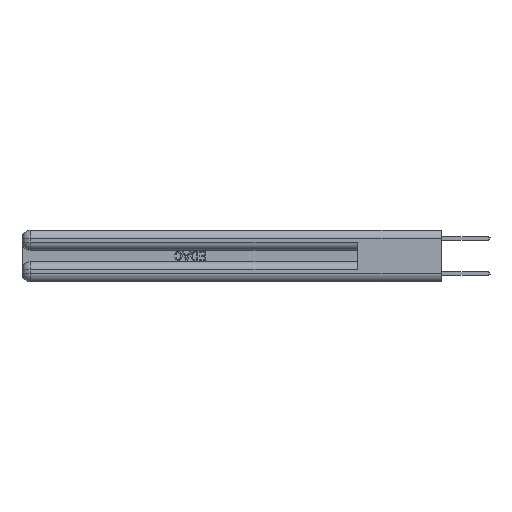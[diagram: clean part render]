
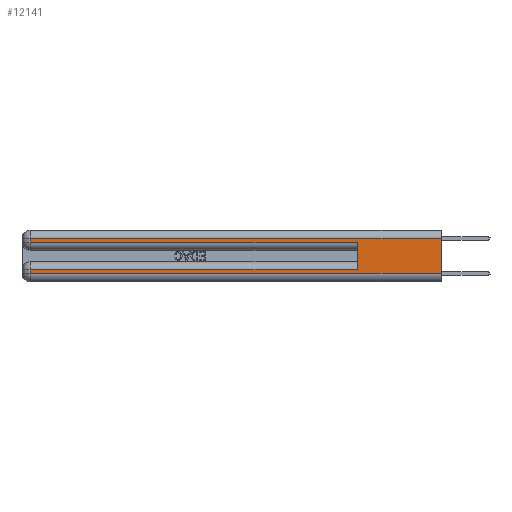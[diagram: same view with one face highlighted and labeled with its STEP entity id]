
A CAD part, left-side view. The second image highlights one B-rep face of the part: STEP entity #12141.
In plain terms, the highlighted planar face has unit normal (-1, 0, 0).
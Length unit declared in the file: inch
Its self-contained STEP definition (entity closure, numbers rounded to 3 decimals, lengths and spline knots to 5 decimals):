
#739 = VECTOR ( 'NONE', #11385, 39.37008 ) ;
#994 = LINE ( 'NONE', #29072, #3283 ) ;
#1477 = CARTESIAN_POINT ( 'NONE',  ( 0., 2.94, 0.06 ) ) ;
#1840 = LINE ( 'NONE', #13558, #28864 ) ;
#2504 = VERTEX_POINT ( 'NONE', #6657 ) ;
#3071 = ORIENTED_EDGE ( 'NONE', *, *, #25304, .F. ) ;
#3097 = VERTEX_POINT ( 'NONE', #22960 ) ;
#3283 = VECTOR ( 'NONE', #17512, 39.37008 ) ;
#3402 = DIRECTION ( 'NONE',  ( 0., -1., 0. ) ) ;
#4942 = ORIENTED_EDGE ( 'NONE', *, *, #20021, .T. ) ;
#6178 = VECTOR ( 'NONE', #18449, 39.37008 ) ;
#6278 = EDGE_CURVE ( 'NONE', #16530, #15183, #1840, .T. ) ;
#6500 = EDGE_CURVE ( 'NONE', #24715, #3097, #994, .T. ) ;
#6657 = CARTESIAN_POINT ( 'NONE',  ( 0., 2.94, 0.285 ) ) ;
#6977 = CARTESIAN_POINT ( 'NONE',  ( 0., 0., 0.31 ) ) ;
#7595 = LINE ( 'NONE', #6977, #22569 ) ;
#8474 = DIRECTION ( 'NONE',  ( 0., 0., -1. ) ) ;
#8587 = VECTOR ( 'NONE', #12057, 39.37008 ) ;
#9437 = ORIENTED_EDGE ( 'NONE', *, *, #24333, .T. ) ;
#10441 = LINE ( 'NONE', #29089, #28031 ) ;
#10533 = VERTEX_POINT ( 'NONE', #13961 ) ;
#11014 = ORIENTED_EDGE ( 'NONE', *, *, #20539, .T. ) ;
#11131 = PLANE ( 'NONE',  #15180 ) ;
#11385 = DIRECTION ( 'NONE',  ( 0., 1., 0. ) ) ;
#11901 = CARTESIAN_POINT ( 'NONE',  ( 0., 2.94, 0.37 ) ) ;
#12056 = VERTEX_POINT ( 'NONE', #30251 ) ;
#12057 = DIRECTION ( 'NONE',  ( 0., 0., -1. ) ) ;
#12141 = ADVANCED_FACE ( 'NONE', ( #16064 ), #11131, .F. ) ;
#12640 = ORIENTED_EDGE ( 'NONE', *, *, #6278, .T. ) ;
#13558 = CARTESIAN_POINT ( 'NONE',  ( 0., 2.94, 0.37 ) ) ;
#13600 = EDGE_CURVE ( 'NONE', #19465, #2504, #16523, .T. ) ;
#13961 = CARTESIAN_POINT ( 'NONE',  ( 0., 0.6, 0.285 ) ) ;
#14319 = LINE ( 'NONE', #28506, #739 ) ;
#15122 = LINE ( 'NONE', #22073, #22269 ) ;
#15180 = AXIS2_PLACEMENT_3D ( 'NONE', #25471, #18680, #18533 ) ;
#15183 = VERTEX_POINT ( 'NONE', #1477 ) ;
#16064 = FACE_OUTER_BOUND ( 'NONE', #29447, .T. ) ;
#16523 = LINE ( 'NONE', #11901, #8587 ) ;
#16530 = VERTEX_POINT ( 'NONE', #20504 ) ;
#16863 = CARTESIAN_POINT ( 'NONE',  ( 0., 0., 0.06 ) ) ;
#17512 = DIRECTION ( 'NONE',  ( 0., 0., -1. ) ) ;
#17768 = EDGE_CURVE ( 'NONE', #2504, #10533, #15122, .T. ) ;
#18066 = CARTESIAN_POINT ( 'NONE',  ( 0., 2.94, 0.31 ) ) ;
#18449 = DIRECTION ( 'NONE',  ( 0., -1., 0. ) ) ;
#18533 = DIRECTION ( 'NONE',  ( 0., 0., -1. ) ) ;
#18577 = ORIENTED_EDGE ( 'NONE', *, *, #6500, .F. ) ;
#18680 = DIRECTION ( 'NONE',  ( 1., 0., 0. ) ) ;
#19465 = VERTEX_POINT ( 'NONE', #18066 ) ;
#20021 = EDGE_CURVE ( 'NONE', #12056, #16530, #14319, .T. ) ;
#20504 = CARTESIAN_POINT ( 'NONE',  ( 0., 2.94, 0.085 ) ) ;
#20539 = EDGE_CURVE ( 'NONE', #15183, #3097, #25388, .T. ) ;
#21697 = ORIENTED_EDGE ( 'NONE', *, *, #17768, .T. ) ;
#22073 = CARTESIAN_POINT ( 'NONE',  ( 0., 0., 0.285 ) ) ;
#22269 = VECTOR ( 'NONE', #3402, 39.37008 ) ;
#22569 = VECTOR ( 'NONE', #23796, 39.37008 ) ;
#22960 = CARTESIAN_POINT ( 'NONE',  ( 0., 0., 0.06 ) ) ;
#23796 = DIRECTION ( 'NONE',  ( 0., 1., 0. ) ) ;
#23915 = CARTESIAN_POINT ( 'NONE',  ( 0., 0., 0.31 ) ) ;
#24333 = EDGE_CURVE ( 'NONE', #24715, #19465, #7595, .T. ) ;
#24715 = VERTEX_POINT ( 'NONE', #23915 ) ;
#25304 = EDGE_CURVE ( 'NONE', #12056, #10533, #10441, .T. ) ;
#25388 = LINE ( 'NONE', #16863, #6178 ) ;
#25471 = CARTESIAN_POINT ( 'NONE',  ( 0., 0., 0.37 ) ) ;
#26916 = DIRECTION ( 'NONE',  ( 0., 0., 1. ) ) ;
#28031 = VECTOR ( 'NONE', #26916, 39.37008 ) ;
#28506 = CARTESIAN_POINT ( 'NONE',  ( 0., 0., 0.085 ) ) ;
#28864 = VECTOR ( 'NONE', #8474, 39.37008 ) ;
#29072 = CARTESIAN_POINT ( 'NONE',  ( 0., 0., 0.37 ) ) ;
#29089 = CARTESIAN_POINT ( 'NONE',  ( 0., 0.6, 0.145 ) ) ;
#29447 = EDGE_LOOP ( 'NONE', ( #18577, #9437, #29465, #21697, #3071, #4942, #12640, #11014 ) ) ;
#29465 = ORIENTED_EDGE ( 'NONE', *, *, #13600, .T. ) ;
#30251 = CARTESIAN_POINT ( 'NONE',  ( 0., 0.6, 0.085 ) ) ;
